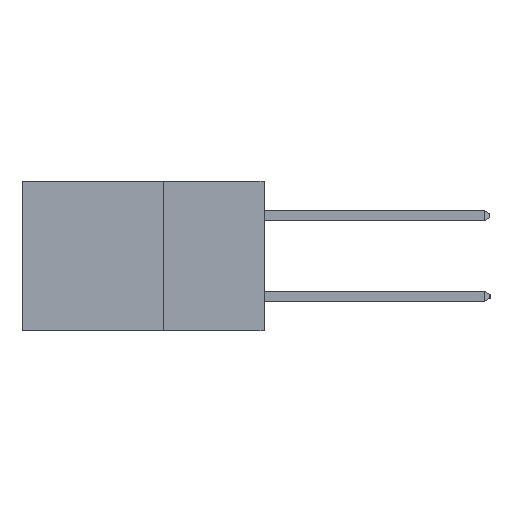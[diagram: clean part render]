
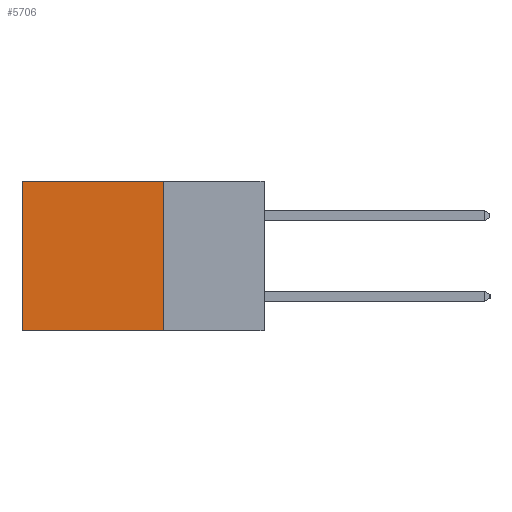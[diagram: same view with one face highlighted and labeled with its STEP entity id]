
A CAD part, left-side view. The second image highlights one B-rep face of the part: STEP entity #5706.
In plain terms, the highlighted planar face has unit normal (-1, 0, 0).
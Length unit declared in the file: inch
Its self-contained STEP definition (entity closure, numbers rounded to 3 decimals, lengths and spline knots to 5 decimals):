
#201 = DIRECTION ( 'NONE',  ( 0., 0., -1. ) ) ;
#669 = CARTESIAN_POINT ( 'NONE',  ( 0.2615, 0.25, -0.37 ) ) ;
#2420 = VECTOR ( 'NONE', #201, 39.37008 ) ;
#3241 = LINE ( 'NONE', #669, #14896 ) ;
#3303 = VECTOR ( 'NONE', #6803, 39.37008 ) ;
#5632 = CARTESIAN_POINT ( 'NONE',  ( 0.2615, 0.6, 0. ) ) ;
#5706 = ADVANCED_FACE ( 'NONE', ( #9325 ), #18002, .F. ) ;
#6803 = DIRECTION ( 'NONE',  ( 0., 0., -1. ) ) ;
#7048 = LINE ( 'NONE', #14666, #3303 ) ;
#7061 = DIRECTION ( 'NONE',  ( 0., 1., 0. ) ) ;
#7114 = ORIENTED_EDGE ( 'NONE', *, *, #12543, .F. ) ;
#8146 = ORIENTED_EDGE ( 'NONE', *, *, #12945, .T. ) ;
#8307 = ORIENTED_EDGE ( 'NONE', *, *, #9464, .T. ) ;
#8315 = EDGE_CURVE ( 'NONE', #8592, #19491, #3241, .T. ) ;
#8552 = CARTESIAN_POINT ( 'NONE',  ( 0.2615, 0.6, -0.37 ) ) ;
#8559 = CARTESIAN_POINT ( 'NONE',  ( 0.2615, 0.25, -0.37 ) ) ;
#8592 = VERTEX_POINT ( 'NONE', #12458 ) ;
#9215 = DIRECTION ( 'NONE',  ( 0., 1., 0. ) ) ;
#9325 = FACE_OUTER_BOUND ( 'NONE', #18998, .T. ) ;
#9340 = ORIENTED_EDGE ( 'NONE', *, *, #8315, .F. ) ;
#9464 = EDGE_CURVE ( 'NONE', #16539, #19491, #15092, .T. ) ;
#10164 = DIRECTION ( 'NONE',  ( 0., 0., -1. ) ) ;
#11751 = VECTOR ( 'NONE', #9215, 39.37008 ) ;
#12458 = CARTESIAN_POINT ( 'NONE',  ( 0.2615, 0.25, -0.37 ) ) ;
#12543 = EDGE_CURVE ( 'NONE', #18925, #8592, #7048, .T. ) ;
#12945 = EDGE_CURVE ( 'NONE', #18925, #16539, #16423, .T. ) ;
#13588 = AXIS2_PLACEMENT_3D ( 'NONE', #8559, #19574, #10164 ) ;
#14666 = CARTESIAN_POINT ( 'NONE',  ( 0.2615, 0.25, -0.37 ) ) ;
#14896 = VECTOR ( 'NONE', #7061, 39.37008 ) ;
#15092 = LINE ( 'NONE', #19220, #2420 ) ;
#15254 = CARTESIAN_POINT ( 'NONE',  ( 0.2615, 0.25, 0. ) ) ;
#15476 = CARTESIAN_POINT ( 'NONE',  ( 0.2615, 0.25, 0. ) ) ;
#16423 = LINE ( 'NONE', #15476, #11751 ) ;
#16539 = VERTEX_POINT ( 'NONE', #5632 ) ;
#18002 = PLANE ( 'NONE',  #13588 ) ;
#18925 = VERTEX_POINT ( 'NONE', #15254 ) ;
#18998 = EDGE_LOOP ( 'NONE', ( #8307, #9340, #7114, #8146 ) ) ;
#19220 = CARTESIAN_POINT ( 'NONE',  ( 0.2615, 0.6, -0.37 ) ) ;
#19491 = VERTEX_POINT ( 'NONE', #8552 ) ;
#19574 = DIRECTION ( 'NONE',  ( 1., 0., 0. ) ) ;
